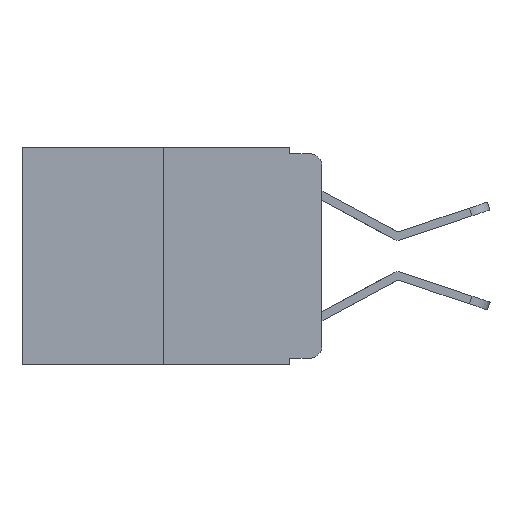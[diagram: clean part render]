
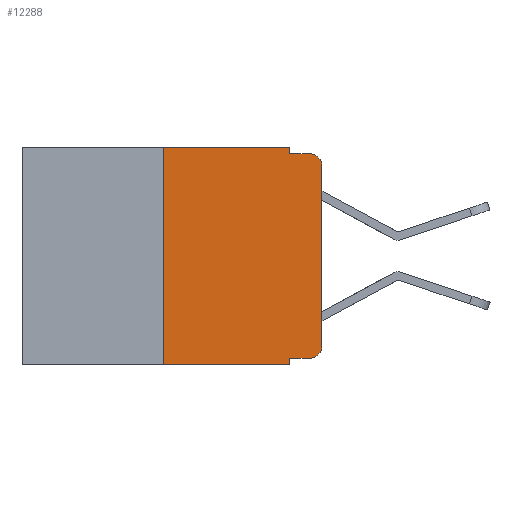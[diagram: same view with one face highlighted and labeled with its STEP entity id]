
A CAD part, left-side view. The second image highlights one B-rep face of the part: STEP entity #12288.
In plain terms, the highlighted planar face has unit normal (-1, 0, 0).
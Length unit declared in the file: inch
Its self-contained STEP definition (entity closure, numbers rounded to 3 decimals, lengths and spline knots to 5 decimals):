
#159 = LINE ( 'NONE', #6408, #8065 ) ;
#393 = DIRECTION ( 'NONE',  ( 0., -1., 0. ) ) ;
#515 = VERTEX_POINT ( 'NONE', #1641 ) ;
#569 = EDGE_CURVE ( 'NONE', #3589, #11766, #11674, .T. ) ;
#610 = CARTESIAN_POINT ( 'NONE',  ( 0., 0.25, 0. ) ) ;
#1138 = VERTEX_POINT ( 'NONE', #12854 ) ;
#1473 = VERTEX_POINT ( 'NONE', #7840 ) ;
#1476 = DIRECTION ( 'NONE',  ( 0., 0., -1. ) ) ;
#1589 = DIRECTION ( 'NONE',  ( 0., 0., 1. ) ) ;
#1622 = CARTESIAN_POINT ( 'NONE',  ( 0., 0.051, 0. ) ) ;
#1641 = CARTESIAN_POINT ( 'NONE',  ( 0., 0.02, -0.01 ) ) ;
#1806 = ORIENTED_EDGE ( 'NONE', *, *, #13329, .F. ) ;
#2136 = CIRCLE ( 'NONE', #10561, 0.02 ) ;
#2217 = CARTESIAN_POINT ( 'NONE',  ( 0., 0.473, -0.343 ) ) ;
#2343 = VERTEX_POINT ( 'NONE', #9436 ) ;
#2467 = VECTOR ( 'NONE', #6665, 39.37008 ) ;
#2593 = AXIS2_PLACEMENT_3D ( 'NONE', #11326, #11380, #9194 ) ;
#2787 = EDGE_CURVE ( 'NONE', #6739, #515, #10381, .T. ) ;
#2977 = ORIENTED_EDGE ( 'NONE', *, *, #8953, .T. ) ;
#3096 = EDGE_CURVE ( 'NONE', #1473, #1138, #11068, .T. ) ;
#3128 = FACE_OUTER_BOUND ( 'NONE', #12898, .T. ) ;
#3370 = CARTESIAN_POINT ( 'NONE',  ( 0., 0.051, -0.01 ) ) ;
#3387 = PLANE ( 'NONE',  #2593 ) ;
#3398 = LINE ( 'NONE', #9368, #8676 ) ;
#3589 = VERTEX_POINT ( 'NONE', #7935 ) ;
#3743 = ORIENTED_EDGE ( 'NONE', *, *, #9748, .T. ) ;
#3767 = CARTESIAN_POINT ( 'NONE',  ( 0., 0.02, -0.313 ) ) ;
#4138 = CARTESIAN_POINT ( 'NONE',  ( 0., 0.051, -0.343 ) ) ;
#4218 = DIRECTION ( 'NONE',  ( -1., 0., 0. ) ) ;
#4390 = ORIENTED_EDGE ( 'NONE', *, *, #8797, .T. ) ;
#4403 = CARTESIAN_POINT ( 'NONE',  ( 0., 0.051, -0.01 ) ) ;
#4409 = VECTOR ( 'NONE', #6783, 39.37008 ) ;
#4822 = CARTESIAN_POINT ( 'NONE',  ( 0., 0.051, -0.333 ) ) ;
#4901 = DIRECTION ( 'NONE',  ( 0., 0., 1. ) ) ;
#5407 = VECTOR ( 'NONE', #8573, 39.37008 ) ;
#5822 = LINE ( 'NONE', #2217, #4409 ) ;
#5867 = ORIENTED_EDGE ( 'NONE', *, *, #2787, .F. ) ;
#5993 = VECTOR ( 'NONE', #9333, 39.37008 ) ;
#6408 = CARTESIAN_POINT ( 'NONE',  ( 0., 0.051, 0. ) ) ;
#6665 = DIRECTION ( 'NONE',  ( 0., -1., 0. ) ) ;
#6739 = VERTEX_POINT ( 'NONE', #3370 ) ;
#6783 = DIRECTION ( 'NONE',  ( 0., -1., 0. ) ) ;
#6847 = VECTOR ( 'NONE', #4901, 39.37008 ) ;
#7626 = EDGE_CURVE ( 'NONE', #11766, #13146, #3398, .T. ) ;
#7840 = CARTESIAN_POINT ( 'NONE',  ( 0., 0., -0.313 ) ) ;
#7912 = ORIENTED_EDGE ( 'NONE', *, *, #7626, .F. ) ;
#7935 = CARTESIAN_POINT ( 'NONE',  ( 0., 0.25, -0.343 ) ) ;
#7984 = VECTOR ( 'NONE', #1589, 39.37008 ) ;
#8065 = VECTOR ( 'NONE', #8678, 39.37008 ) ;
#8141 = CARTESIAN_POINT ( 'NONE',  ( 0., 0.25, 0. ) ) ;
#8388 = EDGE_CURVE ( 'NONE', #1138, #515, #8485, .T. ) ;
#8423 = VERTEX_POINT ( 'NONE', #12091 ) ;
#8485 = CIRCLE ( 'NONE', #13489, 0.02 ) ;
#8573 = DIRECTION ( 'NONE',  ( 0., 0., -1. ) ) ;
#8676 = VECTOR ( 'NONE', #393, 39.37008 ) ;
#8678 = DIRECTION ( 'NONE',  ( 0., 0., -1. ) ) ;
#8797 = EDGE_CURVE ( 'NONE', #3589, #9819, #5822, .T. ) ;
#8953 = EDGE_CURVE ( 'NONE', #8423, #2343, #9343, .T. ) ;
#9194 = DIRECTION ( 'NONE',  ( 0., 0., -1. ) ) ;
#9333 = DIRECTION ( 'NONE',  ( 0., -1., 0. ) ) ;
#9343 = LINE ( 'NONE', #4822, #5993 ) ;
#9368 = CARTESIAN_POINT ( 'NONE',  ( 0., 0.473, 0. ) ) ;
#9436 = CARTESIAN_POINT ( 'NONE',  ( 0., 0.02, -0.333 ) ) ;
#9748 = EDGE_CURVE ( 'NONE', #2343, #1473, #2136, .T. ) ;
#9819 = VERTEX_POINT ( 'NONE', #4138 ) ;
#9832 = CARTESIAN_POINT ( 'NONE',  ( 0., 0.02, -0.03 ) ) ;
#9936 = ORIENTED_EDGE ( 'NONE', *, *, #3096, .T. ) ;
#10184 = ORIENTED_EDGE ( 'NONE', *, *, #8388, .T. ) ;
#10381 = LINE ( 'NONE', #4403, #2467 ) ;
#10528 = ORIENTED_EDGE ( 'NONE', *, *, #13324, .F. ) ;
#10561 = AXIS2_PLACEMENT_3D ( 'NONE', #3767, #13760, #1476 ) ;
#11068 = LINE ( 'NONE', #14018, #6847 ) ;
#11326 = CARTESIAN_POINT ( 'NONE',  ( 0., 0.473, 0. ) ) ;
#11380 = DIRECTION ( 'NONE',  ( 1., 0., 0. ) ) ;
#11674 = LINE ( 'NONE', #610, #7984 ) ;
#11766 = VERTEX_POINT ( 'NONE', #8141 ) ;
#12091 = CARTESIAN_POINT ( 'NONE',  ( 0., 0.051, -0.333 ) ) ;
#12151 = ORIENTED_EDGE ( 'NONE', *, *, #569, .F. ) ;
#12288 = ADVANCED_FACE ( 'NONE', ( #3128 ), #3387, .F. ) ;
#12854 = CARTESIAN_POINT ( 'NONE',  ( 0., 0., -0.03 ) ) ;
#12898 = EDGE_LOOP ( 'NONE', ( #9936, #10184, #5867, #10528, #7912, #12151, #4390, #1806, #2977, #3743 ) ) ;
#13008 = CARTESIAN_POINT ( 'NONE',  ( 0., 0.051, 0. ) ) ;
#13146 = VERTEX_POINT ( 'NONE', #1622 ) ;
#13324 = EDGE_CURVE ( 'NONE', #13146, #6739, #14052, .T. ) ;
#13329 = EDGE_CURVE ( 'NONE', #8423, #9819, #159, .T. ) ;
#13489 = AXIS2_PLACEMENT_3D ( 'NONE', #9832, #4218, #14266 ) ;
#13760 = DIRECTION ( 'NONE',  ( -1., 0., 0. ) ) ;
#14018 = CARTESIAN_POINT ( 'NONE',  ( 0., 0., 0. ) ) ;
#14052 = LINE ( 'NONE', #13008, #5407 ) ;
#14266 = DIRECTION ( 'NONE',  ( 0., 0., -1. ) ) ;
